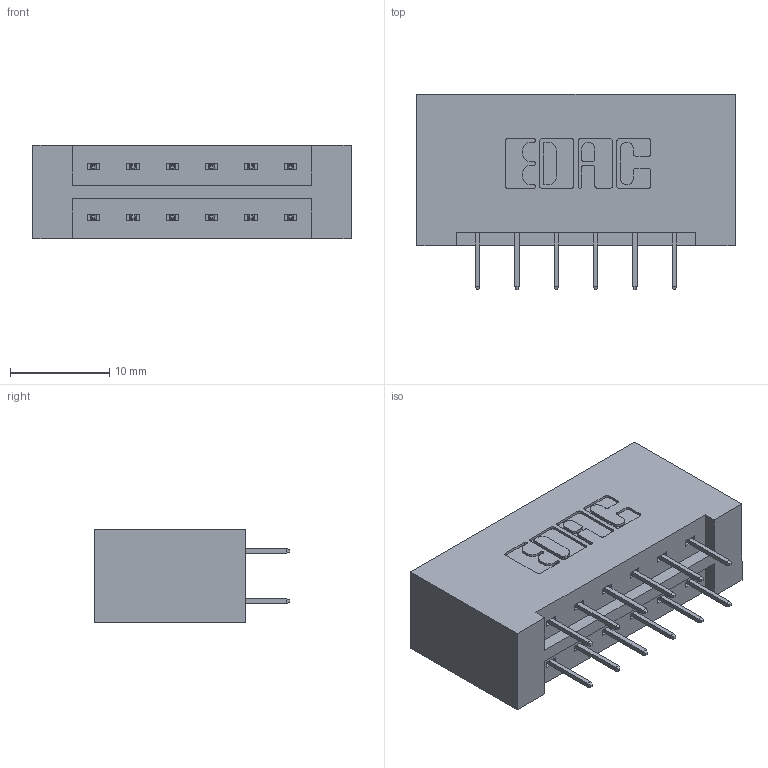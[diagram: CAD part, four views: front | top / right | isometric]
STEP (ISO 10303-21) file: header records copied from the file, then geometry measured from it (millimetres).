
FILE_DESCRIPTION (( 'STEP AP203' ), '1' );
FILE_NAME ('333-012-524-201.STEP', '2018-08-01T00:10:15', ( '' ), ( '' ), 'SwSTEP 2.0', 'SolidWorks 2016', '' );
FILE_SCHEMA (( 'CONFIG_CONTROL_DESIGN' ));
Length unit declared in the file: inch
Products named in the file (3): 333 Part_Lugless; 345-292-001_345-293-124; 333-012-524-201
Assembly tree (13 placements, depth 2):
  333-012-524-201
    333 Part_Lugless
    345-292-001_345-293-124  x12
Bounding box: 32.03 x 19.69 x 9.4 mm (x, y, z)
Volume: 3547.4 mm3; surface area: 3777 mm2
Topology: 13 solids, 13 shells, 778 faces, 2195 edges, 1414 vertices
Faces by surface type: plane 570, cylinder 208
Entity records: 8313 total; most frequent: CARTESIAN_POINT 1418, ORIENTED_EDGE 1354, DIRECTION 1269, EDGE_CURVE 677, LINE 561, VECTOR 561, VERTEX_POINT 446, AXIS2_PLACEMENT_3D 354
